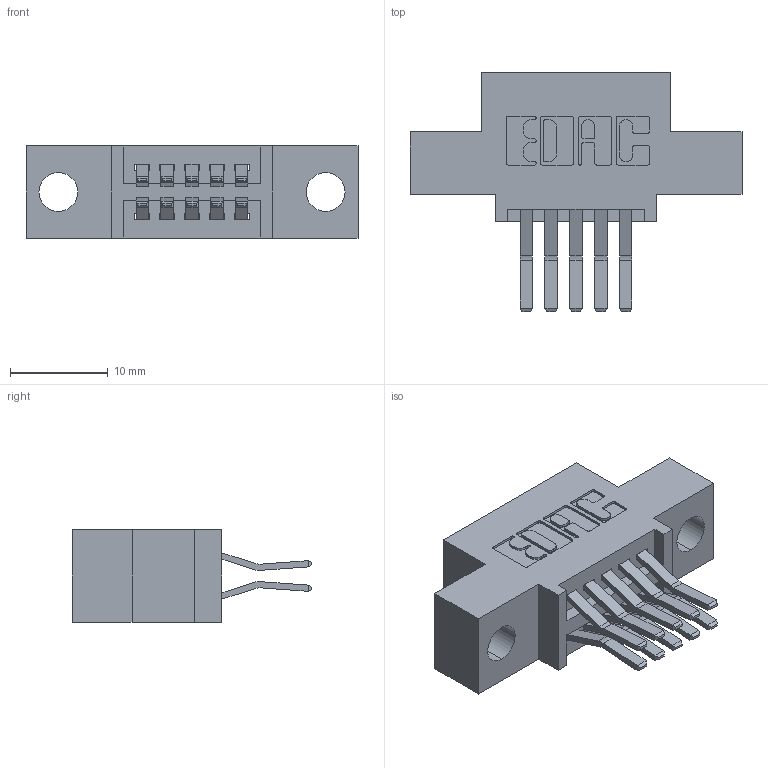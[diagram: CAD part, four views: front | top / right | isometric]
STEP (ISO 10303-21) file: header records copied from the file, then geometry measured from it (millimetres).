
FILE_DESCRIPTION (( 'STEP AP203' ), '1' );
FILE_NAME ('345-010-560-504.STEP', '2021-05-19T15:36:44', ( '' ), ( '' ), 'SwSTEP 2.0', 'SolidWorks 2020', '' );
FILE_SCHEMA (( 'CONFIG_CONTROL_DESIGN' ));
Length unit declared in the file: inch
Products named in the file (3): 345 Part_0.110 Offset - 0.156 Dia-TI; 345-292-001_560 Tail; 345-010-560-504
Assembly tree (11 placements, depth 2):
  345-010-560-504
    345 Part_0.110 Offset - 0.156 Dia-TI
    345-292-001_560 Tail  x10
Bounding box: 33.91 x 24.45 x 9.4 mm (x, y, z)
Volume: 2836.7 mm3; surface area: 3589.6 mm2
Topology: 11 solids, 11 shells, 664 faces, 1939 edges, 1278 vertices
Faces by surface type: plane 428, cylinder 236
Entity records: 9543 total; most frequent: CARTESIAN_POINT 1642, ORIENTED_EDGE 1574, DIRECTION 1495, EDGE_CURVE 787, VECTOR 631, LINE 631, VERTEX_POINT 522, AXIS2_PLACEMENT_3D 432
